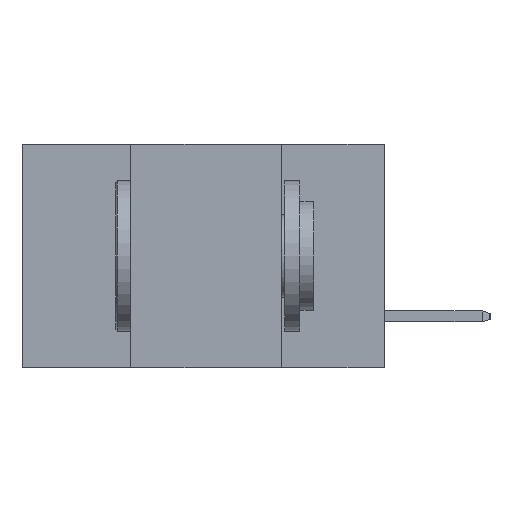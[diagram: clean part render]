
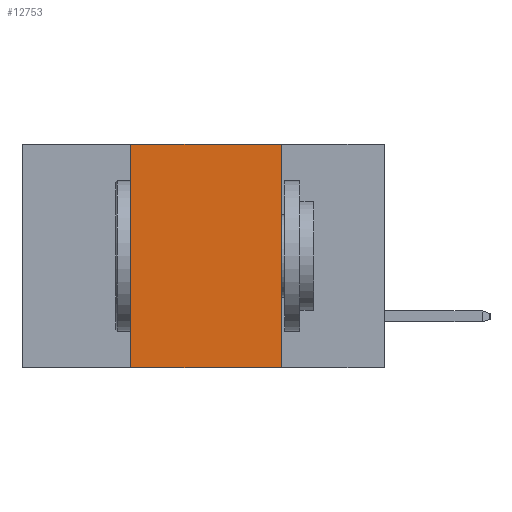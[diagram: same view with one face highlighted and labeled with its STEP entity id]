
A CAD part, left-side view. The second image highlights one B-rep face of the part: STEP entity #12753.
In plain terms, the highlighted planar face has unit normal (-1, 0, 0).
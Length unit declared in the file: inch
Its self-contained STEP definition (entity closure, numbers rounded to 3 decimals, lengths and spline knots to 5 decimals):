
#521 = AXIS2_PLACEMENT_3D ( 'NONE', #24903, #7724, #21208 ) ;
#859 = ORIENTED_EDGE ( 'NONE', *, *, #24699, .F. ) ;
#1219 = VECTOR ( 'NONE', #5335, 39.37008 ) ;
#1379 = CARTESIAN_POINT ( 'NONE',  ( 0., 0.6, -0.37 ) ) ;
#2419 = VECTOR ( 'NONE', #6792, 39.37008 ) ;
#2673 = EDGE_CURVE ( 'NONE', #4395, #25034, #21875, .T. ) ;
#2772 = VECTOR ( 'NONE', #21914, 39.37008 ) ;
#3039 = LINE ( 'NONE', #24080, #2419 ) ;
#4395 = VERTEX_POINT ( 'NONE', #6242 ) ;
#4860 = ORIENTED_EDGE ( 'NONE', *, *, #11219, .F. ) ;
#5126 = CARTESIAN_POINT ( 'NONE',  ( 0., 0.17, 0. ) ) ;
#5327 = EDGE_CURVE ( 'NONE', #4395, #12837, #17571, .T. ) ;
#5335 = DIRECTION ( 'NONE',  ( 0., -1., 0. ) ) ;
#5774 = PLANE ( 'NONE',  #521 ) ;
#6242 = CARTESIAN_POINT ( 'NONE',  ( 0., 0.42, -0.37 ) ) ;
#6384 = FACE_OUTER_BOUND ( 'NONE', #21520, .T. ) ;
#6792 = DIRECTION ( 'NONE',  ( 0., -1., 0. ) ) ;
#7724 = DIRECTION ( 'NONE',  ( 1., 0., 0. ) ) ;
#8854 = ORIENTED_EDGE ( 'NONE', *, *, #2673, .T. ) ;
#9480 = ORIENTED_EDGE ( 'NONE', *, *, #5327, .F. ) ;
#11219 = EDGE_CURVE ( 'NONE', #12837, #19031, #3039, .T. ) ;
#12753 = ADVANCED_FACE ( 'NONE', ( #6384 ), #5774, .F. ) ;
#12837 = VERTEX_POINT ( 'NONE', #13753 ) ;
#13161 = LINE ( 'NONE', #19992, #2772 ) ;
#13753 = CARTESIAN_POINT ( 'NONE',  ( 0., 0.42, 0. ) ) ;
#16961 = VECTOR ( 'NONE', #24595, 39.37008 ) ;
#17571 = LINE ( 'NONE', #24236, #16961 ) ;
#18968 = CARTESIAN_POINT ( 'NONE',  ( 0., 0.17, -0.37 ) ) ;
#19031 = VERTEX_POINT ( 'NONE', #5126 ) ;
#19992 = CARTESIAN_POINT ( 'NONE',  ( 0., 0.17, -0.37 ) ) ;
#21208 = DIRECTION ( 'NONE',  ( 0., 0., -1. ) ) ;
#21520 = EDGE_LOOP ( 'NONE', ( #859, #4860, #9480, #8854 ) ) ;
#21875 = LINE ( 'NONE', #1379, #1219 ) ;
#21914 = DIRECTION ( 'NONE',  ( 0., 0., -1. ) ) ;
#24080 = CARTESIAN_POINT ( 'NONE',  ( 0., 0.6, 0. ) ) ;
#24236 = CARTESIAN_POINT ( 'NONE',  ( 0., 0.42, -0.37 ) ) ;
#24595 = DIRECTION ( 'NONE',  ( 0., 0., 1. ) ) ;
#24699 = EDGE_CURVE ( 'NONE', #19031, #25034, #13161, .T. ) ;
#24903 = CARTESIAN_POINT ( 'NONE',  ( 0., 0.6, 0. ) ) ;
#25034 = VERTEX_POINT ( 'NONE', #18968 ) ;
